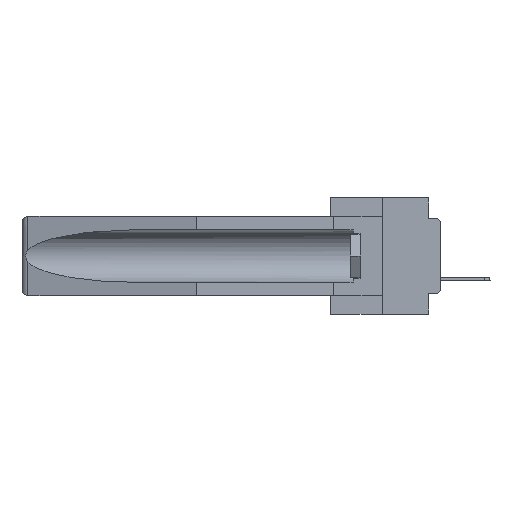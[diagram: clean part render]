
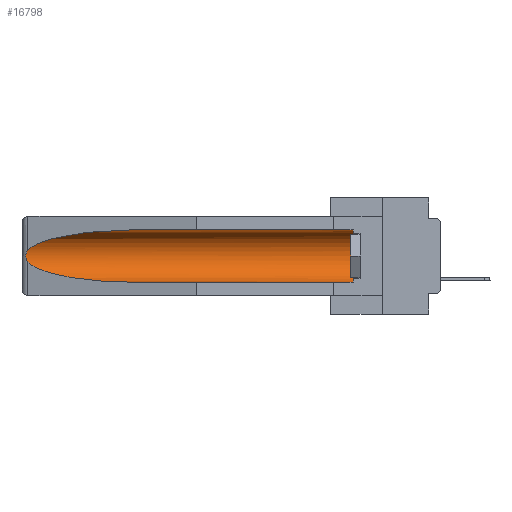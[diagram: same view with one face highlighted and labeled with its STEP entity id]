
A CAD part, left-side view. The second image highlights one B-rep face of the part: STEP entity #16798.
In plain terms, the highlighted cylindrical face has radius 2.857 mm (diameter 5.715 mm), a partial arc.
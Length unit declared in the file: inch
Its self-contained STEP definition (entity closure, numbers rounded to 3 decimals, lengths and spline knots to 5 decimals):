
#270 = B_SPLINE_CURVE_WITH_KNOTS ( 'NONE', 3,
 ( #27704, #11603, #11848, #30404, #25394, #831, #14424, #27586, #24891, #16795 ),
 .UNSPECIFIED., .F., .F.,
 ( 4, 2, 2, 2, 4 ),
 ( 0., 0.00029, 0.00058, 0.00087, 0.00117 ),
 .UNSPECIFIED. ) ;
#347 = CARTESIAN_POINT ( 'NONE',  ( 0.155, -0.30754, -0.059 ) ) ;
#831 = CARTESIAN_POINT ( 'NONE',  ( 0.2675, 1.53308, -0.17534 ) ) ;
#1700 = CARTESIAN_POINT ( 'NONE',  ( 0.26537, 1.52718, -0.14972 ) ) ;
#3798 = DIRECTION ( 'NONE',  ( 0., 0., 1. ) ) ;
#4373 = VERTEX_POINT ( 'NONE', #19728 ) ;
#4702 = VECTOR ( 'NONE', #27428, 39.37008 ) ;
#5488 = VECTOR ( 'NONE', #6629, 39.37008 ) ;
#6073 = CARTESIAN_POINT ( 'NONE',  ( 0.21114, 1.30732, -0.059 ) ) ;
#6086 = CARTESIAN_POINT ( 'NONE',  ( 0.155, 1.07973, -0.059 ) ) ;
#6368 = VERTEX_POINT ( 'NONE', #29498 ) ;
#6629 = DIRECTION ( 'NONE',  ( 0., 1., 0. ) ) ;
#7652 = EDGE_LOOP ( 'NONE', ( #32274, #17934, #25069, #19605, #20672, #17561 ) ) ;
#7744 = CIRCLE ( 'NONE', #29759, 0.1125 ) ;
#8816 = LINE ( 'NONE', #9349, #5488 ) ;
#9054 = DIRECTION ( 'NONE',  ( 0., -1., 0. ) ) ;
#9283 =( BOUNDED_CURVE ( )  B_SPLINE_CURVE ( 3, ( #10321, #15748, #22100, #9561 ),
 .UNSPECIFIED., .F., .F. ) 
 B_SPLINE_CURVE_WITH_KNOTS ( ( 4, 4 ),
 ( 0.1948, 1.5708 ),
 .UNSPECIFIED. ) 
 CURVE ( )  GEOMETRIC_REPRESENTATION_ITEM ( )  RATIONAL_B_SPLINE_CURVE ( ( 1., 0.848, 0.848, 1. ) ) 
 REPRESENTATION_ITEM ( '' )  );
#9349 = CARTESIAN_POINT ( 'NONE',  ( 0.155, -0.30754, -0.284 ) ) ;
#9473 = EDGE_CURVE ( 'NONE', #31186, #29235, #270, .T. ) ;
#9561 = CARTESIAN_POINT ( 'NONE',  ( 0.155, 1.07973, -0.284 ) ) ;
#10321 = CARTESIAN_POINT ( 'NONE',  ( 0.26537, 1.52718, -0.19328 ) ) ;
#11603 = CARTESIAN_POINT ( 'NONE',  ( 0.26597, 1.52961, -0.15275 ) ) ;
#11848 = CARTESIAN_POINT ( 'NONE',  ( 0.26654, 1.53092, -0.15636 ) ) ;
#11982 = EDGE_CURVE ( 'NONE', #6368, #19596, #8816, .T. ) ;
#12215 = VERTEX_POINT ( 'NONE', #6086 ) ;
#12341 = FACE_OUTER_BOUND ( 'NONE', #7652, .T. ) ;
#14027 = CARTESIAN_POINT ( 'NONE',  ( 0.26537, 1.52718, -0.14972 ) ) ;
#14337 = CARTESIAN_POINT ( 'NONE',  ( 0.155, 0.126, -0.1715 ) ) ;
#14424 = CARTESIAN_POINT ( 'NONE',  ( 0.2673, 1.53269, -0.17917 ) ) ;
#15748 = CARTESIAN_POINT ( 'NONE',  ( 0.25451, 1.48313, -0.24835 ) ) ;
#16178 = CYLINDRICAL_SURFACE ( 'NONE', #24246, 0.1125 ) ;
#16795 = CARTESIAN_POINT ( 'NONE',  ( 0.26537, 1.52718, -0.19328 ) ) ;
#16798 = ADVANCED_FACE ( 'NONE', ( #12341 ), #16178, .F. ) ;
#17561 = ORIENTED_EDGE ( 'NONE', *, *, #19463, .T. ) ;
#17934 = ORIENTED_EDGE ( 'NONE', *, *, #9473, .T. ) ;
#19463 = EDGE_CURVE ( 'NONE', #4373, #12215, #27749, .T. ) ;
#19596 = VERTEX_POINT ( 'NONE', #34164 ) ;
#19605 = ORIENTED_EDGE ( 'NONE', *, *, #11982, .F. ) ;
#19728 = CARTESIAN_POINT ( 'NONE',  ( 0.155, 0.126, -0.059 ) ) ;
#20672 = ORIENTED_EDGE ( 'NONE', *, *, #31080, .T. ) ;
#21041 = EDGE_CURVE ( 'NONE', #12215, #31186, #24334, .T. ) ;
#22030 = CARTESIAN_POINT ( 'NONE',  ( 0.155, -0.30754, -0.1715 ) ) ;
#22100 = CARTESIAN_POINT ( 'NONE',  ( 0.21114, 1.30732, -0.284 ) ) ;
#22138 = CARTESIAN_POINT ( 'NONE',  ( 0.25451, 1.48313, -0.09465 ) ) ;
#22378 = DIRECTION ( 'NONE',  ( 0., 1., 0. ) ) ;
#24246 = AXIS2_PLACEMENT_3D ( 'NONE', #22030, #22378, #33209 ) ;
#24334 =( BOUNDED_CURVE ( )  B_SPLINE_CURVE ( 3, ( #24855, #6073, #22138, #14027 ),
 .UNSPECIFIED., .F., .F. ) 
 B_SPLINE_CURVE_WITH_KNOTS ( ( 4, 4 ),
 ( 4.71239, 6.08839 ),
 .UNSPECIFIED. ) 
 CURVE ( )  GEOMETRIC_REPRESENTATION_ITEM ( )  RATIONAL_B_SPLINE_CURVE ( ( 1., 0.848, 0.848, 1. ) ) 
 REPRESENTATION_ITEM ( '' )  );
#24855 = CARTESIAN_POINT ( 'NONE',  ( 0.155, 1.07973, -0.059 ) ) ;
#24891 = CARTESIAN_POINT ( 'NONE',  ( 0.26597, 1.5296, -0.19026 ) ) ;
#25069 = ORIENTED_EDGE ( 'NONE', *, *, #26783, .T. ) ;
#25394 = CARTESIAN_POINT ( 'NONE',  ( 0.2675, 1.53308, -0.16763 ) ) ;
#26783 = EDGE_CURVE ( 'NONE', #29235, #19596, #9283, .T. ) ;
#27428 = DIRECTION ( 'NONE',  ( 0., 1., 0. ) ) ;
#27586 = CARTESIAN_POINT ( 'NONE',  ( 0.26655, 1.53094, -0.18657 ) ) ;
#27704 = CARTESIAN_POINT ( 'NONE',  ( 0.26537, 1.52718, -0.14972 ) ) ;
#27749 = LINE ( 'NONE', #347, #4702 ) ;
#29235 = VERTEX_POINT ( 'NONE', #33009 ) ;
#29498 = CARTESIAN_POINT ( 'NONE',  ( 0.155, 0.126, -0.284 ) ) ;
#29759 = AXIS2_PLACEMENT_3D ( 'NONE', #14337, #9054, #3798 ) ;
#30404 = CARTESIAN_POINT ( 'NONE',  ( 0.2673, 1.5327, -0.16383 ) ) ;
#31080 = EDGE_CURVE ( 'NONE', #6368, #4373, #7744, .T. ) ;
#31186 = VERTEX_POINT ( 'NONE', #1700 ) ;
#32274 = ORIENTED_EDGE ( 'NONE', *, *, #21041, .T. ) ;
#33009 = CARTESIAN_POINT ( 'NONE',  ( 0.26537, 1.52718, -0.19328 ) ) ;
#33209 = DIRECTION ( 'NONE',  ( 0., 0., 1. ) ) ;
#34164 = CARTESIAN_POINT ( 'NONE',  ( 0.155, 1.07973, -0.284 ) ) ;
